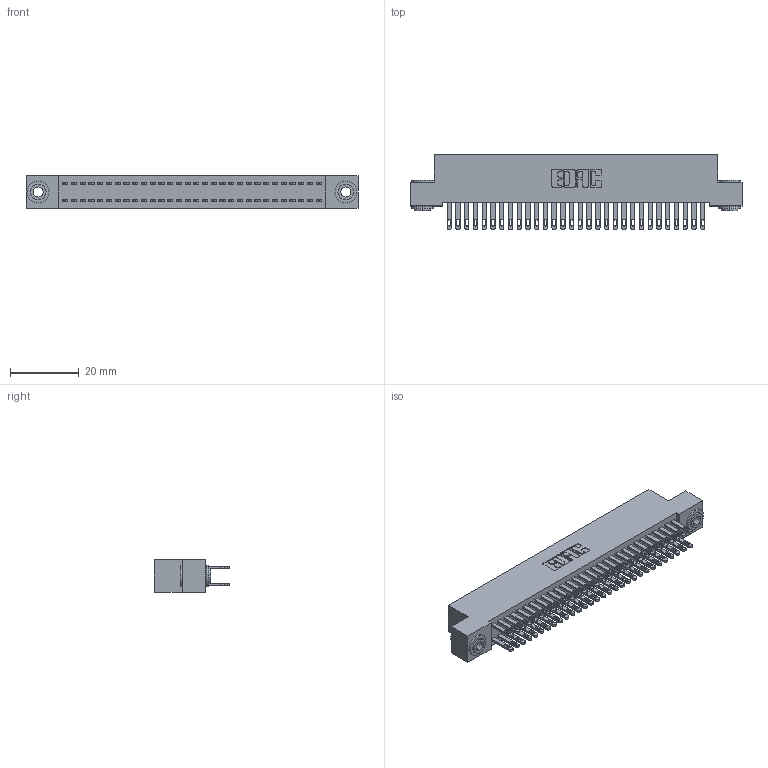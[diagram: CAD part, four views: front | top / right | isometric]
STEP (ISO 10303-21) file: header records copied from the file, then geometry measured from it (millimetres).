
FILE_DESCRIPTION (( 'STEP AP203' ), '1' );
FILE_NAME ('892-060-500-203.STEP', '2020-09-21T19:08:36', ( '' ), ( '' ), 'SwSTEP 2.0', 'SolidWorks 2020', '' );
FILE_SCHEMA (( 'CONFIG_CONTROL_DESIGN' ));
Length unit declared in the file: inch
Products named in the file (4): 842 Part_.156 TH; 892-060-500-203; 342-250-002_345-250-002-102; 345-292-001_345-293-100
Assembly tree (63 placements, depth 2):
  892-060-500-203
    842 Part_.156 TH
    345-292-001_345-293-100  x60
    342-250-002_345-250-002-102  x2
Bounding box: 96.52 x 21.85 x 9.4 mm (x, y, z)
Volume: 8821.7 mm3; surface area: 14852.3 mm2
Topology: 63 solids, 63 shells, 3028 faces, 9195 edges, 6126 vertices
Faces by surface type: plane 1876, cylinder 1144, cone 8
Entity records: 21300 total; most frequent: CARTESIAN_POINT 3517, ORIENTED_EDGE 3446, DIRECTION 3061, EDGE_CURVE 1723, VECTOR 1567, LINE 1567, VERTEX_POINT 1146, AXIS2_PLACEMENT_3D 747
